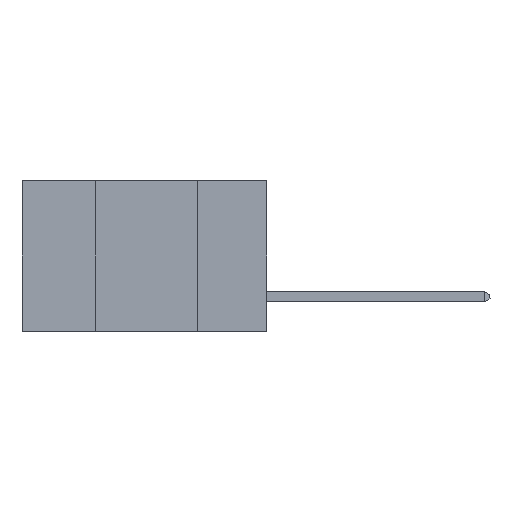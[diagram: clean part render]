
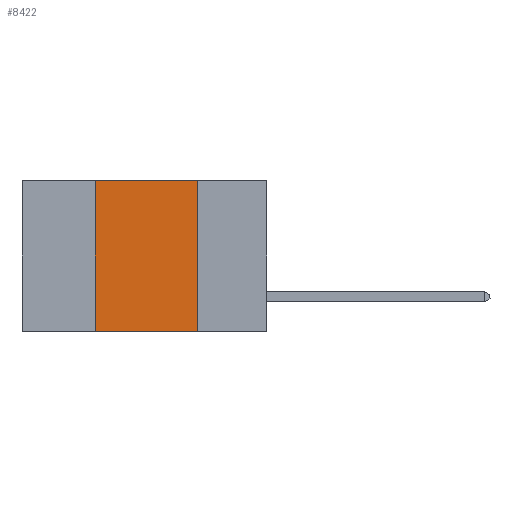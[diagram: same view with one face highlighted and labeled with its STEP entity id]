
A CAD part, left-side view. The second image highlights one B-rep face of the part: STEP entity #8422.
In plain terms, the highlighted planar face has unit normal (-1, 0, 0).
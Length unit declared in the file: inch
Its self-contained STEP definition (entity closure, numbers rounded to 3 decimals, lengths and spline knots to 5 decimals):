
#39 = ORIENTED_EDGE ( 'NONE', *, *, #7351, .T. ) ;
#712 = ORIENTED_EDGE ( 'NONE', *, *, #4914, .F. ) ;
#836 = EDGE_CURVE ( 'NONE', #860, #9744, #866, .T. ) ;
#860 = VERTEX_POINT ( 'NONE', #2669 ) ;
#866 = LINE ( 'NONE', #1710, #5454 ) ;
#1160 = PLANE ( 'NONE',  #6437 ) ;
#1385 = DIRECTION ( 'NONE',  ( 0., 0., -1. ) ) ;
#1710 = CARTESIAN_POINT ( 'NONE',  ( 0., 0.6, 0. ) ) ;
#2074 = ORIENTED_EDGE ( 'NONE', *, *, #836, .F. ) ;
#2235 = VECTOR ( 'NONE', #5516, 39.37008 ) ;
#2504 = LINE ( 'NONE', #4590, #2235 ) ;
#2522 = DIRECTION ( 'NONE',  ( 0., -1., 0. ) ) ;
#2669 = CARTESIAN_POINT ( 'NONE',  ( 0., 0.42, 0. ) ) ;
#2736 = DIRECTION ( 'NONE',  ( 0., 0., -1. ) ) ;
#3109 = FACE_OUTER_BOUND ( 'NONE', #10225, .T. ) ;
#3675 = CARTESIAN_POINT ( 'NONE',  ( 0., 0.6, -0.37 ) ) ;
#4201 = CARTESIAN_POINT ( 'NONE',  ( 0., 0.17, -0.37 ) ) ;
#4523 = CARTESIAN_POINT ( 'NONE',  ( 0., 0.6, 0. ) ) ;
#4542 = VERTEX_POINT ( 'NONE', #7390 ) ;
#4590 = CARTESIAN_POINT ( 'NONE',  ( 0., 0.42, 0. ) ) ;
#4756 = ORIENTED_EDGE ( 'NONE', *, *, #10642, .F. ) ;
#4914 = EDGE_CURVE ( 'NONE', #9744, #10276, #9450, .T. ) ;
#5454 = VECTOR ( 'NONE', #10641, 39.37008 ) ;
#5516 = DIRECTION ( 'NONE',  ( 0., 0., 1. ) ) ;
#5806 = LINE ( 'NONE', #3675, #7844 ) ;
#6329 = DIRECTION ( 'NONE',  ( 1., 0., 0. ) ) ;
#6437 = AXIS2_PLACEMENT_3D ( 'NONE', #4523, #6329, #2736 ) ;
#7351 = EDGE_CURVE ( 'NONE', #4542, #10276, #5806, .T. ) ;
#7390 = CARTESIAN_POINT ( 'NONE',  ( 0., 0.42, -0.37 ) ) ;
#7447 = VECTOR ( 'NONE', #1385, 39.37008 ) ;
#7844 = VECTOR ( 'NONE', #2522, 39.37008 ) ;
#8422 = ADVANCED_FACE ( 'NONE', ( #3109 ), #1160, .F. ) ;
#9072 = CARTESIAN_POINT ( 'NONE',  ( 0., 0.17, 0. ) ) ;
#9450 = LINE ( 'NONE', #9746, #7447 ) ;
#9744 = VERTEX_POINT ( 'NONE', #9072 ) ;
#9746 = CARTESIAN_POINT ( 'NONE',  ( 0., 0.17, 0. ) ) ;
#10225 = EDGE_LOOP ( 'NONE', ( #712, #2074, #4756, #39 ) ) ;
#10276 = VERTEX_POINT ( 'NONE', #4201 ) ;
#10641 = DIRECTION ( 'NONE',  ( 0., -1., 0. ) ) ;
#10642 = EDGE_CURVE ( 'NONE', #4542, #860, #2504, .T. ) ;
